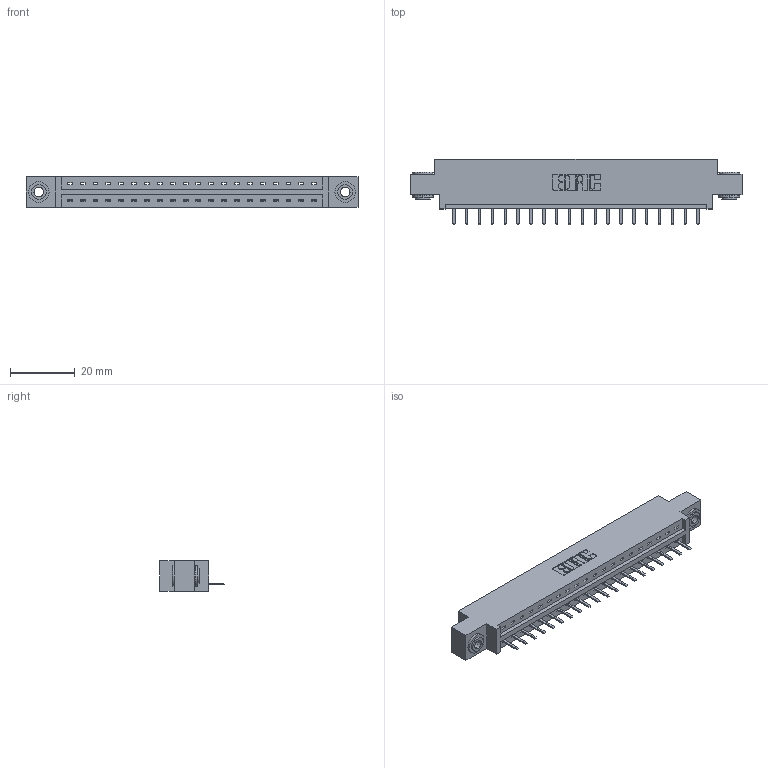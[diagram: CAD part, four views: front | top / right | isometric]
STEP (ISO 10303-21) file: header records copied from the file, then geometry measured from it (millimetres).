
FILE_DESCRIPTION (( 'STEP AP203' ), '1' );
FILE_NAME ('387-020-520-603.STEP', '2019-10-02T22:05:47', ( '' ), ( '' ), 'SwSTEP 2.0', 'SolidWorks 2016', '' );
FILE_SCHEMA (( 'CONFIG_CONTROL_DESIGN' ));
Length unit declared in the file: inch
Products named in the file (4): 345-250-002_345-250-002-102; 337 Part_0.170 Offset - 0.156 Dia-TH; 345-292-001_345-293-120; 387-020-520-603
Assembly tree (23 placements, depth 2):
  387-020-520-603
    337 Part_0.170 Offset - 0.156 Dia-TH
    345-292-001_345-293-120  x20
    345-250-002_345-250-002-102  x2
Bounding box: 102.26 x 20.02 x 9.4 mm (x, y, z)
Volume: 10197.3 mm3; surface area: 10537.3 mm2
Topology: 23 solids, 23 shells, 1476 faces, 4319 edges, 2822 vertices
Faces by surface type: plane 1044, cylinder 424, cone 8
Entity records: 18608 total; most frequent: CARTESIAN_POINT 3229, ORIENTED_EDGE 3166, DIRECTION 2785, EDGE_CURVE 1583, LINE 1427, VECTOR 1427, VERTEX_POINT 1050, AXIS2_PLACEMENT_3D 679
